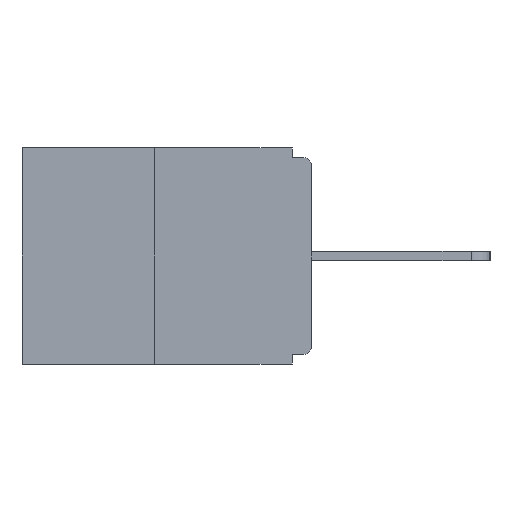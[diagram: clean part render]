
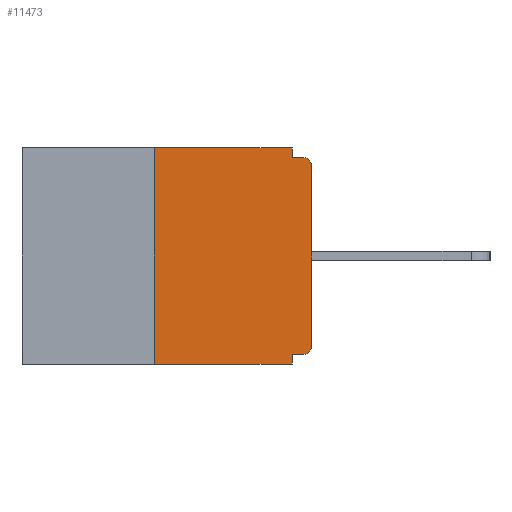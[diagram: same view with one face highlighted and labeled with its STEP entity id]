
A CAD part, left-side view. The second image highlights one B-rep face of the part: STEP entity #11473.
In plain terms, the highlighted planar face has unit normal (-1, 0, 0).
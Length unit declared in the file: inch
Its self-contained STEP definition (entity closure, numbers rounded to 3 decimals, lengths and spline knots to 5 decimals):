
#2 = VECTOR ( 'NONE', #1051, 39.37008 ) ;
#1051 = DIRECTION ( 'NONE',  ( 0., -1., 0. ) ) ;
#1072 = VECTOR ( 'NONE', #12167, 39.37008 ) ;
#1308 = DIRECTION ( 'NONE',  ( 0., 0., 1. ) ) ;
#1926 = PLANE ( 'NONE',  #1964 ) ;
#1964 = AXIS2_PLACEMENT_3D ( 'NONE', #15832, #11797, #7501 ) ;
#1968 = CARTESIAN_POINT ( 'NONE',  ( 0., 0.015, -0.313 ) ) ;
#2063 = DIRECTION ( 'NONE',  ( 0., 0., -1. ) ) ;
#2219 = ORIENTED_EDGE ( 'NONE', *, *, #16038, .T. ) ;
#2228 = ORIENTED_EDGE ( 'NONE', *, *, #14939, .T. ) ;
#2300 = VERTEX_POINT ( 'NONE', #5822 ) ;
#2578 = CARTESIAN_POINT ( 'NONE',  ( 0., 0.46, -0.343 ) ) ;
#2672 = EDGE_CURVE ( 'NONE', #11955, #12993, #4978, .T. ) ;
#2745 = LINE ( 'NONE', #9711, #14758 ) ;
#2795 = VERTEX_POINT ( 'NONE', #15240 ) ;
#3472 = CARTESIAN_POINT ( 'NONE',  ( 0., 0., -0.313 ) ) ;
#3512 = ORIENTED_EDGE ( 'NONE', *, *, #6506, .F. ) ;
#4252 = EDGE_CURVE ( 'NONE', #7842, #14357, #7805, .T. ) ;
#4451 = ORIENTED_EDGE ( 'NONE', *, *, #4252, .F. ) ;
#4843 = ORIENTED_EDGE ( 'NONE', *, *, #12539, .F. ) ;
#4978 = LINE ( 'NONE', #9212, #2 ) ;
#5125 = CARTESIAN_POINT ( 'NONE',  ( 0., 0., -0.328 ) ) ;
#5481 = CARTESIAN_POINT ( 'NONE',  ( 0., 0.031, -0.343 ) ) ;
#5510 = LINE ( 'NONE', #9562, #11577 ) ;
#5822 = CARTESIAN_POINT ( 'NONE',  ( 0., 0.25, -0.343 ) ) ;
#5829 = EDGE_CURVE ( 'NONE', #2300, #11955, #12313, .T. ) ;
#5910 = DIRECTION ( 'NONE',  ( -1., 0., 0. ) ) ;
#6506 = EDGE_CURVE ( 'NONE', #13452, #7618, #8401, .T. ) ;
#6933 = CARTESIAN_POINT ( 'NONE',  ( 0., 0., -0.015 ) ) ;
#7294 = EDGE_CURVE ( 'NONE', #2795, #15680, #15322, .T. ) ;
#7373 = CARTESIAN_POINT ( 'NONE',  ( 0., 0., -0.03 ) ) ;
#7501 = DIRECTION ( 'NONE',  ( 0., 0., -1. ) ) ;
#7511 = AXIS2_PLACEMENT_3D ( 'NONE', #15541, #5910, #10315 ) ;
#7618 = VERTEX_POINT ( 'NONE', #17223 ) ;
#7805 = LINE ( 'NONE', #12196, #9450 ) ;
#7842 = VERTEX_POINT ( 'NONE', #7880 ) ;
#7880 = CARTESIAN_POINT ( 'NONE',  ( 0., 0.031, -0.328 ) ) ;
#8323 = ORIENTED_EDGE ( 'NONE', *, *, #5829, .F. ) ;
#8401 = LINE ( 'NONE', #6933, #15006 ) ;
#9212 = CARTESIAN_POINT ( 'NONE',  ( 0., 0.46, 0. ) ) ;
#9450 = VECTOR ( 'NONE', #13552, 39.37008 ) ;
#9562 = CARTESIAN_POINT ( 'NONE',  ( 0., 0., 0. ) ) ;
#9711 = CARTESIAN_POINT ( 'NONE',  ( 0., 0.031, 0. ) ) ;
#10315 = DIRECTION ( 'NONE',  ( 0., 0., -1. ) ) ;
#10900 = VECTOR ( 'NONE', #12034, 39.37008 ) ;
#10942 = EDGE_LOOP ( 'NONE', ( #13089, #8323, #15221, #4451, #4843, #16675, #2228, #2219, #3512, #15484 ) ) ;
#11137 = VERTEX_POINT ( 'NONE', #7373 ) ;
#11473 = ADVANCED_FACE ( 'NONE', ( #13182 ), #1926, .F. ) ;
#11577 = VECTOR ( 'NONE', #1308, 39.37008 ) ;
#11797 = DIRECTION ( 'NONE',  ( 1., 0., 0. ) ) ;
#11955 = VERTEX_POINT ( 'NONE', #11962 ) ;
#11962 = CARTESIAN_POINT ( 'NONE',  ( 0., 0.25, 0. ) ) ;
#12005 = LINE ( 'NONE', #5125, #12433 ) ;
#12034 = DIRECTION ( 'NONE',  ( 0., 0., 1. ) ) ;
#12072 = LINE ( 'NONE', #2578, #1072 ) ;
#12167 = DIRECTION ( 'NONE',  ( 0., -1., 0. ) ) ;
#12196 = CARTESIAN_POINT ( 'NONE',  ( 0., 0.031, -0.343 ) ) ;
#12313 = LINE ( 'NONE', #13490, #10900 ) ;
#12433 = VECTOR ( 'NONE', #16294, 39.37008 ) ;
#12539 = EDGE_CURVE ( 'NONE', #2795, #7842, #12005, .T. ) ;
#12993 = VERTEX_POINT ( 'NONE', #13869 ) ;
#13089 = ORIENTED_EDGE ( 'NONE', *, *, #2672, .F. ) ;
#13182 = FACE_OUTER_BOUND ( 'NONE', #10942, .T. ) ;
#13452 = VERTEX_POINT ( 'NONE', #15686 ) ;
#13490 = CARTESIAN_POINT ( 'NONE',  ( 0., 0.25, 0. ) ) ;
#13552 = DIRECTION ( 'NONE',  ( 0., 0., -1. ) ) ;
#13791 = DIRECTION ( 'NONE',  ( 0., -1., 0. ) ) ;
#13869 = CARTESIAN_POINT ( 'NONE',  ( 0., 0.031, 0. ) ) ;
#14004 = DIRECTION ( 'NONE',  ( 0., 0., -1. ) ) ;
#14171 = AXIS2_PLACEMENT_3D ( 'NONE', #1968, #14589, #2063 ) ;
#14267 = EDGE_CURVE ( 'NONE', #12993, #13452, #2745, .T. ) ;
#14357 = VERTEX_POINT ( 'NONE', #5481 ) ;
#14589 = DIRECTION ( 'NONE',  ( -1., 0., 0. ) ) ;
#14758 = VECTOR ( 'NONE', #14004, 39.37008 ) ;
#14939 = EDGE_CURVE ( 'NONE', #15680, #11137, #5510, .T. ) ;
#15006 = VECTOR ( 'NONE', #13791, 39.37008 ) ;
#15221 = ORIENTED_EDGE ( 'NONE', *, *, #15439, .T. ) ;
#15240 = CARTESIAN_POINT ( 'NONE',  ( 0., 0.015, -0.328 ) ) ;
#15322 = CIRCLE ( 'NONE', #14171, 0.015 ) ;
#15439 = EDGE_CURVE ( 'NONE', #2300, #14357, #12072, .T. ) ;
#15484 = ORIENTED_EDGE ( 'NONE', *, *, #14267, .F. ) ;
#15541 = CARTESIAN_POINT ( 'NONE',  ( 0., 0.015, -0.03 ) ) ;
#15680 = VERTEX_POINT ( 'NONE', #3472 ) ;
#15686 = CARTESIAN_POINT ( 'NONE',  ( 0., 0.031, -0.015 ) ) ;
#15832 = CARTESIAN_POINT ( 'NONE',  ( 0., 0.46, 0. ) ) ;
#16038 = EDGE_CURVE ( 'NONE', #11137, #7618, #18016, .T. ) ;
#16294 = DIRECTION ( 'NONE',  ( 0., 1., 0. ) ) ;
#16675 = ORIENTED_EDGE ( 'NONE', *, *, #7294, .T. ) ;
#17223 = CARTESIAN_POINT ( 'NONE',  ( 0., 0.015, -0.015 ) ) ;
#18016 = CIRCLE ( 'NONE', #7511, 0.015 ) ;
